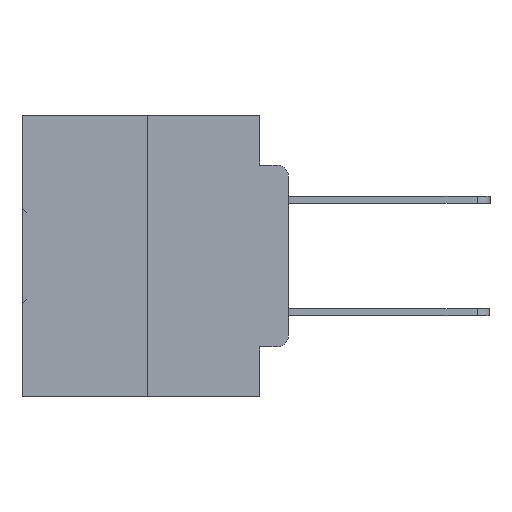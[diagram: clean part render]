
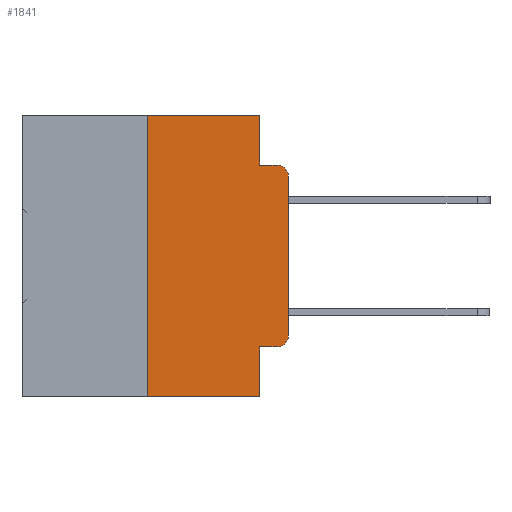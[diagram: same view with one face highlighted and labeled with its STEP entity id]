
A CAD part, left-side view. The second image highlights one B-rep face of the part: STEP entity #1841.
In plain terms, the highlighted planar face has unit normal (-1, 0, 0).
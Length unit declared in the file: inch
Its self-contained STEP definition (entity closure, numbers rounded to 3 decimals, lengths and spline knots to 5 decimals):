
#111 = DIRECTION ( 'NONE',  ( 0., -1., 0. ) ) ;
#982 = DIRECTION ( 'NONE',  ( 0., -1., 0. ) ) ;
#1049 = CARTESIAN_POINT ( 'NONE',  ( 0., 0., 0. ) ) ;
#1136 = EDGE_CURVE ( 'NONE', #28574, #28928, #33732, .T. ) ;
#1512 = DIRECTION ( 'NONE',  ( 0., -1., 0. ) ) ;
#1841 = ADVANCED_FACE ( 'NONE', ( #24939 ), #17550, .F. ) ;
#2215 = DIRECTION ( 'NONE',  ( 1., 0., 0. ) ) ;
#2759 = CARTESIAN_POINT ( 'NONE',  ( 0., 0.25, 0. ) ) ;
#4173 = LINE ( 'NONE', #23788, #17388 ) ;
#4280 = CARTESIAN_POINT ( 'NONE',  ( 0., 0.051, -0.4115 ) ) ;
#4482 = CARTESIAN_POINT ( 'NONE',  ( 0., 0.473, 0. ) ) ;
#4885 = EDGE_LOOP ( 'NONE', ( #22983, #28252, #15581, #19241, #26182, #25524, #25657, #25775, #25365, #24479 ) ) ;
#5726 = LINE ( 'NONE', #2759, #32617 ) ;
#5808 = VECTOR ( 'NONE', #6654, 39.37008 ) ;
#6654 = DIRECTION ( 'NONE',  ( 0., 0., -1. ) ) ;
#7136 = CARTESIAN_POINT ( 'NONE',  ( 0., 0.02, -0.0885 ) ) ;
#8659 = EDGE_CURVE ( 'NONE', #28928, #19050, #32599, .T. ) ;
#9916 = EDGE_CURVE ( 'NONE', #14549, #30319, #24549, .T. ) ;
#11211 = DIRECTION ( 'NONE',  ( -1., 0., 0. ) ) ;
#11436 = EDGE_CURVE ( 'NONE', #15234, #14549, #13390, .T. ) ;
#11705 = CARTESIAN_POINT ( 'NONE',  ( 0., 0.25, -0.5 ) ) ;
#12588 = VECTOR ( 'NONE', #25444, 39.37008 ) ;
#13377 = AXIS2_PLACEMENT_3D ( 'NONE', #30771, #15262, #33285 ) ;
#13390 = LINE ( 'NONE', #17552, #12588 ) ;
#13630 = EDGE_CURVE ( 'NONE', #25822, #26184, #4173, .T. ) ;
#13767 = CARTESIAN_POINT ( 'NONE',  ( 0., 0.051, -0.4115 ) ) ;
#14536 = EDGE_CURVE ( 'NONE', #27103, #30319, #31886, .T. ) ;
#14549 = VERTEX_POINT ( 'NONE', #25650 ) ;
#15234 = VERTEX_POINT ( 'NONE', #28634 ) ;
#15262 = DIRECTION ( 'NONE',  ( -1., 0., 0. ) ) ;
#15581 = ORIENTED_EDGE ( 'NONE', *, *, #9916, .F. ) ;
#15806 = CARTESIAN_POINT ( 'NONE',  ( 0., 0.051, -0.5 ) ) ;
#16066 = EDGE_CURVE ( 'NONE', #25822, #25620, #5726, .T. ) ;
#17388 = VECTOR ( 'NONE', #111, 39.37008 ) ;
#17550 = PLANE ( 'NONE',  #30314 ) ;
#17552 = CARTESIAN_POINT ( 'NONE',  ( 0., 0.051, 0. ) ) ;
#18315 = CARTESIAN_POINT ( 'NONE',  ( 0., 0., -0.3915 ) ) ;
#18725 = VECTOR ( 'NONE', #29848, 39.37008 ) ;
#19050 = VERTEX_POINT ( 'NONE', #18315 ) ;
#19241 = ORIENTED_EDGE ( 'NONE', *, *, #11436, .F. ) ;
#19358 = EDGE_CURVE ( 'NONE', #19050, #27103, #26460, .T. ) ;
#19861 = LINE ( 'NONE', #30161, #5808 ) ;
#20123 = VECTOR ( 'NONE', #1512, 39.37008 ) ;
#20199 = EDGE_CURVE ( 'NONE', #25620, #15234, #24061, .T. ) ;
#21345 = CARTESIAN_POINT ( 'NONE',  ( 0., 0.25, 0. ) ) ;
#21354 = DIRECTION ( 'NONE',  ( 0., 0., 1. ) ) ;
#22918 = DIRECTION ( 'NONE',  ( 0., -1., 0. ) ) ;
#22983 = ORIENTED_EDGE ( 'NONE', *, *, #19358, .T. ) ;
#23558 = AXIS2_PLACEMENT_3D ( 'NONE', #26847, #11211, #29405 ) ;
#23788 = CARTESIAN_POINT ( 'NONE',  ( 0., 0.473, -0.5 ) ) ;
#24061 = LINE ( 'NONE', #4482, #30870 ) ;
#24479 = ORIENTED_EDGE ( 'NONE', *, *, #8659, .T. ) ;
#24549 = LINE ( 'NONE', #32311, #29771 ) ;
#24754 = CARTESIAN_POINT ( 'NONE',  ( 0., 0.02, -0.4115 ) ) ;
#24939 = FACE_OUTER_BOUND ( 'NONE', #4885, .T. ) ;
#25365 = ORIENTED_EDGE ( 'NONE', *, *, #1136, .T. ) ;
#25444 = DIRECTION ( 'NONE',  ( 0., 0., -1. ) ) ;
#25524 = ORIENTED_EDGE ( 'NONE', *, *, #16066, .F. ) ;
#25620 = VERTEX_POINT ( 'NONE', #21345 ) ;
#25650 = CARTESIAN_POINT ( 'NONE',  ( 0., 0.051, -0.0885 ) ) ;
#25657 = ORIENTED_EDGE ( 'NONE', *, *, #13630, .T. ) ;
#25775 = ORIENTED_EDGE ( 'NONE', *, *, #33330, .F. ) ;
#25822 = VERTEX_POINT ( 'NONE', #11705 ) ;
#26182 = ORIENTED_EDGE ( 'NONE', *, *, #20199, .F. ) ;
#26184 = VERTEX_POINT ( 'NONE', #15806 ) ;
#26460 = LINE ( 'NONE', #1049, #18725 ) ;
#26847 = CARTESIAN_POINT ( 'NONE',  ( 0., 0.02, -0.3915 ) ) ;
#27103 = VERTEX_POINT ( 'NONE', #29570 ) ;
#28252 = ORIENTED_EDGE ( 'NONE', *, *, #14536, .T. ) ;
#28574 = VERTEX_POINT ( 'NONE', #4280 ) ;
#28634 = CARTESIAN_POINT ( 'NONE',  ( 0., 0.051, 0. ) ) ;
#28928 = VERTEX_POINT ( 'NONE', #24754 ) ;
#29405 = DIRECTION ( 'NONE',  ( 0., 0., -1. ) ) ;
#29570 = CARTESIAN_POINT ( 'NONE',  ( 0., 0., -0.1085 ) ) ;
#29771 = VECTOR ( 'NONE', #982, 39.37008 ) ;
#29848 = DIRECTION ( 'NONE',  ( 0., 0., 1. ) ) ;
#29964 = CARTESIAN_POINT ( 'NONE',  ( 0., 0.473, 0. ) ) ;
#30034 = DIRECTION ( 'NONE',  ( 0., 0., -1. ) ) ;
#30161 = CARTESIAN_POINT ( 'NONE',  ( 0., 0.051, 0. ) ) ;
#30314 = AXIS2_PLACEMENT_3D ( 'NONE', #29964, #2215, #30034 ) ;
#30319 = VERTEX_POINT ( 'NONE', #7136 ) ;
#30771 = CARTESIAN_POINT ( 'NONE',  ( 0., 0.02, -0.1085 ) ) ;
#30870 = VECTOR ( 'NONE', #22918, 39.37008 ) ;
#31886 = CIRCLE ( 'NONE', #13377, 0.02 ) ;
#32311 = CARTESIAN_POINT ( 'NONE',  ( 0., 0.051, -0.0885 ) ) ;
#32599 = CIRCLE ( 'NONE', #23558, 0.02 ) ;
#32617 = VECTOR ( 'NONE', #21354, 39.37008 ) ;
#33285 = DIRECTION ( 'NONE',  ( 0., 0., -1. ) ) ;
#33330 = EDGE_CURVE ( 'NONE', #28574, #26184, #19861, .T. ) ;
#33732 = LINE ( 'NONE', #13767, #20123 ) ;
